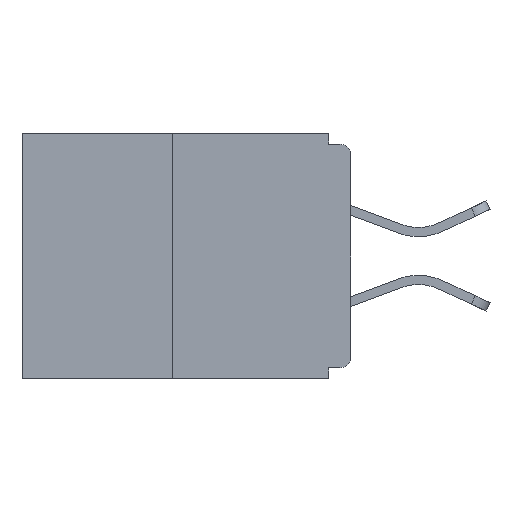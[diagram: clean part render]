
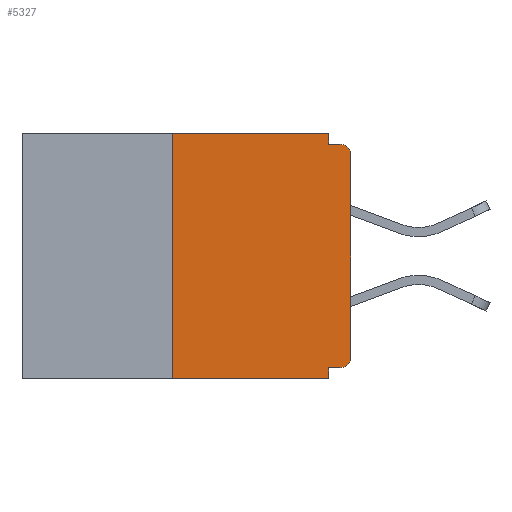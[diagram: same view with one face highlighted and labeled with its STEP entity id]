
A CAD part, left-side view. The second image highlights one B-rep face of the part: STEP entity #5327.
In plain terms, the highlighted planar face has unit normal (-1, 0, 0).
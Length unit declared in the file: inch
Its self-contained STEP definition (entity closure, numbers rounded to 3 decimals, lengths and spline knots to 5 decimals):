
#60 = CARTESIAN_POINT ( 'NONE',  ( 0., 0.015, -0.03 ) ) ;
#107 = CARTESIAN_POINT ( 'NONE',  ( 0., 0.25, 0. ) ) ;
#313 = EDGE_CURVE ( 'NONE', #8282, #3555, #17227, .T. ) ;
#818 = DIRECTION ( 'NONE',  ( 0., -1., 0. ) ) ;
#1247 = ORIENTED_EDGE ( 'NONE', *, *, #8119, .T. ) ;
#1352 = CARTESIAN_POINT ( 'NONE',  ( 0., 0., -0.313 ) ) ;
#1549 = VECTOR ( 'NONE', #11132, 39.37008 ) ;
#2260 = VERTEX_POINT ( 'NONE', #8459 ) ;
#2626 = AXIS2_PLACEMENT_3D ( 'NONE', #60, #12334, #20896 ) ;
#2866 = DIRECTION ( 'NONE',  ( 1., 0., 0. ) ) ;
#3328 = VERTEX_POINT ( 'NONE', #21794 ) ;
#3555 = VERTEX_POINT ( 'NONE', #107 ) ;
#3745 = EDGE_CURVE ( 'NONE', #6684, #16891, #17335, .T. ) ;
#3834 = ORIENTED_EDGE ( 'NONE', *, *, #8390, .F. ) ;
#3912 = DIRECTION ( 'NONE',  ( 0., 0., -1. ) ) ;
#4200 = VECTOR ( 'NONE', #8306, 39.37008 ) ;
#4320 = CARTESIAN_POINT ( 'NONE',  ( 0., 0.25, -0.343 ) ) ;
#5104 = LINE ( 'NONE', #13590, #14682 ) ;
#5277 = EDGE_CURVE ( 'NONE', #11208, #9539, #17782, .T. ) ;
#5327 = ADVANCED_FACE ( 'NONE', ( #7369 ), #13584, .F. ) ;
#5524 = CARTESIAN_POINT ( 'NONE',  ( 0., 0.015, -0.313 ) ) ;
#5561 = LINE ( 'NONE', #11933, #4200 ) ;
#6015 = CARTESIAN_POINT ( 'NONE',  ( 0., 0., 0. ) ) ;
#6641 = CARTESIAN_POINT ( 'NONE',  ( 0., 0.25, 0. ) ) ;
#6684 = VERTEX_POINT ( 'NONE', #12086 ) ;
#7369 = FACE_OUTER_BOUND ( 'NONE', #21481, .T. ) ;
#7959 = CARTESIAN_POINT ( 'NONE',  ( 0., 0.46, -0.343 ) ) ;
#8095 = CIRCLE ( 'NONE', #22597, 0.015 ) ;
#8119 = EDGE_CURVE ( 'NONE', #18588, #3328, #17426, .T. ) ;
#8282 = VERTEX_POINT ( 'NONE', #4320 ) ;
#8306 = DIRECTION ( 'NONE',  ( 0., 1., 0. ) ) ;
#8380 = DIRECTION ( 'NONE',  ( 0., 0., 1. ) ) ;
#8390 = EDGE_CURVE ( 'NONE', #18673, #11208, #5104, .T. ) ;
#8459 = CARTESIAN_POINT ( 'NONE',  ( 0., 0.015, -0.328 ) ) ;
#9338 = EDGE_CURVE ( 'NONE', #8282, #16891, #10069, .T. ) ;
#9539 = VERTEX_POINT ( 'NONE', #18933 ) ;
#9717 = DIRECTION ( 'NONE',  ( 0., -1., 0. ) ) ;
#9868 = CARTESIAN_POINT ( 'NONE',  ( 0., 0.46, 0. ) ) ;
#10032 = CARTESIAN_POINT ( 'NONE',  ( 0., 0.031, -0.015 ) ) ;
#10069 = LINE ( 'NONE', #7959, #13956 ) ;
#10070 = EDGE_CURVE ( 'NONE', #2260, #18588, #8095, .T. ) ;
#10727 = EDGE_CURVE ( 'NONE', #3555, #18673, #21217, .T. ) ;
#10991 = CARTESIAN_POINT ( 'NONE',  ( 0., 0.46, 0. ) ) ;
#11132 = DIRECTION ( 'NONE',  ( 0., 0., 1. ) ) ;
#11208 = VERTEX_POINT ( 'NONE', #10032 ) ;
#11585 = DIRECTION ( 'NONE',  ( 0., 0., -1. ) ) ;
#11933 = CARTESIAN_POINT ( 'NONE',  ( 0., 0., -0.328 ) ) ;
#12086 = CARTESIAN_POINT ( 'NONE',  ( 0., 0.031, -0.328 ) ) ;
#12334 = DIRECTION ( 'NONE',  ( -1., 0., 0. ) ) ;
#12549 = VECTOR ( 'NONE', #8380, 39.37008 ) ;
#12759 = EDGE_CURVE ( 'NONE', #2260, #6684, #5561, .T. ) ;
#13418 = DIRECTION ( 'NONE',  ( 0., 0., -1. ) ) ;
#13484 = ORIENTED_EDGE ( 'NONE', *, *, #9338, .T. ) ;
#13584 = PLANE ( 'NONE',  #14196 ) ;
#13590 = CARTESIAN_POINT ( 'NONE',  ( 0., 0.031, 0. ) ) ;
#13956 = VECTOR ( 'NONE', #9717, 39.37008 ) ;
#14196 = AXIS2_PLACEMENT_3D ( 'NONE', #9868, #2866, #13418 ) ;
#14417 = EDGE_CURVE ( 'NONE', #3328, #9539, #22189, .T. ) ;
#14682 = VECTOR ( 'NONE', #16774, 39.37008 ) ;
#14715 = CARTESIAN_POINT ( 'NONE',  ( 0., 0.031, 0. ) ) ;
#16569 = VECTOR ( 'NONE', #18102, 39.37008 ) ;
#16629 = CARTESIAN_POINT ( 'NONE',  ( 0., 0.031, -0.343 ) ) ;
#16774 = DIRECTION ( 'NONE',  ( 0., 0., -1. ) ) ;
#16891 = VERTEX_POINT ( 'NONE', #17314 ) ;
#17227 = LINE ( 'NONE', #6641, #12549 ) ;
#17314 = CARTESIAN_POINT ( 'NONE',  ( 0., 0.031, -0.343 ) ) ;
#17335 = LINE ( 'NONE', #16629, #22536 ) ;
#17426 = LINE ( 'NONE', #6015, #1549 ) ;
#17782 = LINE ( 'NONE', #18220, #19431 ) ;
#18102 = DIRECTION ( 'NONE',  ( 0., -1., 0. ) ) ;
#18220 = CARTESIAN_POINT ( 'NONE',  ( 0., 0., -0.015 ) ) ;
#18588 = VERTEX_POINT ( 'NONE', #1352 ) ;
#18673 = VERTEX_POINT ( 'NONE', #14715 ) ;
#18933 = CARTESIAN_POINT ( 'NONE',  ( 0., 0.015, -0.015 ) ) ;
#19430 = DIRECTION ( 'NONE',  ( -1., 0., 0. ) ) ;
#19431 = VECTOR ( 'NONE', #818, 39.37008 ) ;
#19444 = ORIENTED_EDGE ( 'NONE', *, *, #10070, .T. ) ;
#20044 = ORIENTED_EDGE ( 'NONE', *, *, #3745, .F. ) ;
#20896 = DIRECTION ( 'NONE',  ( 0., 0., -1. ) ) ;
#21204 = ORIENTED_EDGE ( 'NONE', *, *, #5277, .F. ) ;
#21217 = LINE ( 'NONE', #10991, #16569 ) ;
#21481 = EDGE_LOOP ( 'NONE', ( #22571, #22115, #13484, #20044, #22275, #19444, #1247, #22573, #21204, #3834 ) ) ;
#21794 = CARTESIAN_POINT ( 'NONE',  ( 0., 0., -0.03 ) ) ;
#22115 = ORIENTED_EDGE ( 'NONE', *, *, #313, .F. ) ;
#22189 = CIRCLE ( 'NONE', #2626, 0.015 ) ;
#22275 = ORIENTED_EDGE ( 'NONE', *, *, #12759, .F. ) ;
#22536 = VECTOR ( 'NONE', #11585, 39.37008 ) ;
#22571 = ORIENTED_EDGE ( 'NONE', *, *, #10727, .F. ) ;
#22573 = ORIENTED_EDGE ( 'NONE', *, *, #14417, .T. ) ;
#22597 = AXIS2_PLACEMENT_3D ( 'NONE', #5524, #19430, #3912 ) ;
